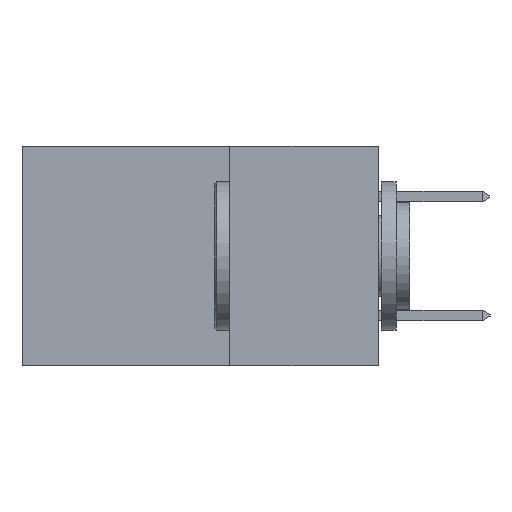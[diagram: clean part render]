
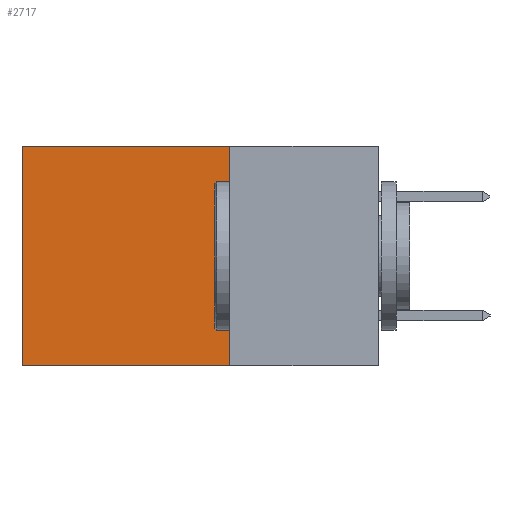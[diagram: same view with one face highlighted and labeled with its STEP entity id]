
A CAD part, left-side view. The second image highlights one B-rep face of the part: STEP entity #2717.
In plain terms, the highlighted planar face has unit normal (-1, 0, 0).
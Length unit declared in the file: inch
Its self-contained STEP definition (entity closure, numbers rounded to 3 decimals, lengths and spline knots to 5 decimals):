
#465 = LINE ( 'NONE', #12008, #17406 ) ;
#905 = DIRECTION ( 'NONE',  ( 0., 1., 0. ) ) ;
#1346 = VERTEX_POINT ( 'NONE', #1951 ) ;
#1951 = CARTESIAN_POINT ( 'NONE',  ( 0.2615, 0.6, -0.37 ) ) ;
#2596 = LINE ( 'NONE', #11361, #11534 ) ;
#2717 = ADVANCED_FACE ( 'NONE', ( #18787 ), #11811, .F. ) ;
#2794 = VERTEX_POINT ( 'NONE', #3626 ) ;
#3454 = DIRECTION ( 'NONE',  ( 0., 1., 0. ) ) ;
#3626 = CARTESIAN_POINT ( 'NONE',  ( 0.2615, 0.6, 0. ) ) ;
#4660 = EDGE_CURVE ( 'NONE', #11151, #13076, #8191, .T. ) ;
#5938 = CARTESIAN_POINT ( 'NONE',  ( 0.2615, 0.25, 0. ) ) ;
#6140 = EDGE_CURVE ( 'NONE', #13076, #1346, #465, .T. ) ;
#7860 = CARTESIAN_POINT ( 'NONE',  ( 0.2615, 0.6, -0.37 ) ) ;
#8191 = LINE ( 'NONE', #14913, #20444 ) ;
#8820 = EDGE_LOOP ( 'NONE', ( #15170, #13404, #11874, #15122 ) ) ;
#9192 = AXIS2_PLACEMENT_3D ( 'NONE', #11374, #11239, #11027 ) ;
#9453 = DIRECTION ( 'NONE',  ( 0., 0., -1. ) ) ;
#11027 = DIRECTION ( 'NONE',  ( 0., 0., -1. ) ) ;
#11151 = VERTEX_POINT ( 'NONE', #5938 ) ;
#11239 = DIRECTION ( 'NONE',  ( 1., 0., 0. ) ) ;
#11361 = CARTESIAN_POINT ( 'NONE',  ( 0.2615, 0.25, 0. ) ) ;
#11374 = CARTESIAN_POINT ( 'NONE',  ( 0.2615, 0.25, -0.37 ) ) ;
#11534 = VECTOR ( 'NONE', #3454, 39.37008 ) ;
#11811 = PLANE ( 'NONE',  #9192 ) ;
#11874 = ORIENTED_EDGE ( 'NONE', *, *, #4660, .F. ) ;
#12008 = CARTESIAN_POINT ( 'NONE',  ( 0.2615, 0.25, -0.37 ) ) ;
#13057 = EDGE_CURVE ( 'NONE', #2794, #1346, #14069, .T. ) ;
#13076 = VERTEX_POINT ( 'NONE', #19064 ) ;
#13404 = ORIENTED_EDGE ( 'NONE', *, *, #6140, .F. ) ;
#14069 = LINE ( 'NONE', #7860, #17840 ) ;
#14411 = EDGE_CURVE ( 'NONE', #11151, #2794, #2596, .T. ) ;
#14832 = DIRECTION ( 'NONE',  ( 0., 0., -1. ) ) ;
#14913 = CARTESIAN_POINT ( 'NONE',  ( 0.2615, 0.25, -0.37 ) ) ;
#15122 = ORIENTED_EDGE ( 'NONE', *, *, #14411, .T. ) ;
#15170 = ORIENTED_EDGE ( 'NONE', *, *, #13057, .T. ) ;
#17406 = VECTOR ( 'NONE', #905, 39.37008 ) ;
#17840 = VECTOR ( 'NONE', #9453, 39.37008 ) ;
#18787 = FACE_OUTER_BOUND ( 'NONE', #8820, .T. ) ;
#19064 = CARTESIAN_POINT ( 'NONE',  ( 0.2615, 0.25, -0.37 ) ) ;
#20444 = VECTOR ( 'NONE', #14832, 39.37008 ) ;
